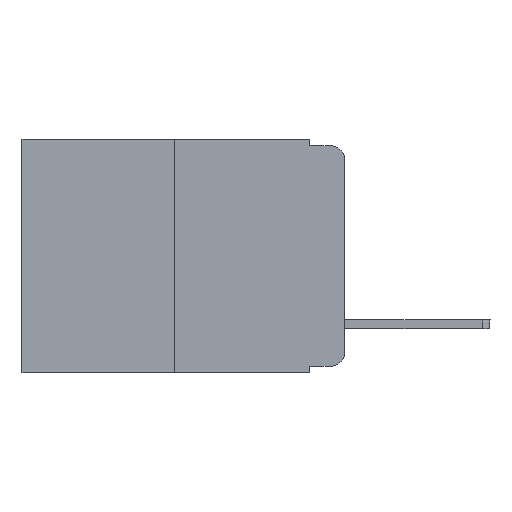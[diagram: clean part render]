
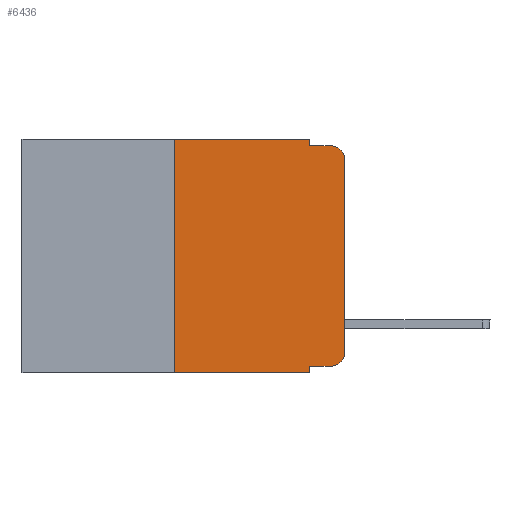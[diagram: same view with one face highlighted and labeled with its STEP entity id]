
A CAD part, left-side view. The second image highlights one B-rep face of the part: STEP entity #6436.
In plain terms, the highlighted planar face has unit normal (-1, 0, 0).
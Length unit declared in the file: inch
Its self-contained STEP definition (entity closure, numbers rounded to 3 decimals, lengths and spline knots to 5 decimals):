
#295 = LINE ( 'NONE', #18152, #21118 ) ;
#316 = VECTOR ( 'NONE', #17345, 39.37008 ) ;
#908 = VERTEX_POINT ( 'NONE', #2108 ) ;
#1001 = ORIENTED_EDGE ( 'NONE', *, *, #9225, .T. ) ;
#1073 = EDGE_CURVE ( 'NONE', #2855, #908, #17449, .T. ) ;
#1702 = DIRECTION ( 'NONE',  ( 0., -1., 0. ) ) ;
#1844 = VECTOR ( 'NONE', #20724, 39.37008 ) ;
#1947 = DIRECTION ( 'NONE',  ( 0., -1., 0. ) ) ;
#2108 = CARTESIAN_POINT ( 'NONE',  ( 0., 0.02, -0.333 ) ) ;
#2473 = CARTESIAN_POINT ( 'NONE',  ( 0., 0., -0.03 ) ) ;
#2579 = ORIENTED_EDGE ( 'NONE', *, *, #15121, .F. ) ;
#2637 = CARTESIAN_POINT ( 'NONE',  ( 0., 0.051, 0. ) ) ;
#2855 = VERTEX_POINT ( 'NONE', #9663 ) ;
#3003 = DIRECTION ( 'NONE',  ( 0., 0., -1. ) ) ;
#3525 = VECTOR ( 'NONE', #1947, 39.37008 ) ;
#3633 = AXIS2_PLACEMENT_3D ( 'NONE', #6027, #19022, #9798 ) ;
#4241 = LINE ( 'NONE', #8364, #20992 ) ;
#4399 = LINE ( 'NONE', #23824, #7563 ) ;
#4755 = EDGE_CURVE ( 'NONE', #8837, #4920, #20600, .T. ) ;
#4906 = EDGE_LOOP ( 'NONE', ( #14602, #11863, #21933, #11710, #2579, #14333, #6421, #10864, #15119, #1001 ) ) ;
#4920 = VERTEX_POINT ( 'NONE', #11579 ) ;
#4939 = DIRECTION ( 'NONE',  ( 0., 0., 1. ) ) ;
#5621 = EDGE_CURVE ( 'NONE', #19535, #14723, #4399, .T. ) ;
#6027 = CARTESIAN_POINT ( 'NONE',  ( 0., 0.02, -0.03 ) ) ;
#6421 = ORIENTED_EDGE ( 'NONE', *, *, #5621, .T. ) ;
#6436 = ADVANCED_FACE ( 'NONE', ( #19042 ), #17907, .F. ) ;
#6632 = CARTESIAN_POINT ( 'NONE',  ( 0., 0.051, 0. ) ) ;
#6854 = DIRECTION ( 'NONE',  ( 0., 0., 1. ) ) ;
#7078 = CARTESIAN_POINT ( 'NONE',  ( 0., 0.473, 0. ) ) ;
#7441 = CARTESIAN_POINT ( 'NONE',  ( 0., 0.051, -0.01 ) ) ;
#7563 = VECTOR ( 'NONE', #1702, 39.37008 ) ;
#7900 = VERTEX_POINT ( 'NONE', #21560 ) ;
#7903 = CARTESIAN_POINT ( 'NONE',  ( 0., 0.051, -0.333 ) ) ;
#7922 = CARTESIAN_POINT ( 'NONE',  ( 0., 0.051, 0. ) ) ;
#8364 = CARTESIAN_POINT ( 'NONE',  ( 0., 0.25, 0. ) ) ;
#8837 = VERTEX_POINT ( 'NONE', #15466 ) ;
#9062 = EDGE_CURVE ( 'NONE', #19535, #14202, #4241, .T. ) ;
#9225 = EDGE_CURVE ( 'NONE', #908, #7900, #19522, .T. ) ;
#9314 = CIRCLE ( 'NONE', #3633, 0.02 ) ;
#9467 = DIRECTION ( 'NONE',  ( 0., -1., 0. ) ) ;
#9663 = CARTESIAN_POINT ( 'NONE',  ( 0., 0.051, -0.333 ) ) ;
#9734 = CARTESIAN_POINT ( 'NONE',  ( 0., 0.051, -0.343 ) ) ;
#9798 = DIRECTION ( 'NONE',  ( 0., 0., -1. ) ) ;
#10069 = EDGE_CURVE ( 'NONE', #22306, #8837, #16290, .T. ) ;
#10257 = VECTOR ( 'NONE', #3003, 39.37008 ) ;
#10864 = ORIENTED_EDGE ( 'NONE', *, *, #21099, .F. ) ;
#11579 = CARTESIAN_POINT ( 'NONE',  ( 0., 0.02, -0.01 ) ) ;
#11710 = ORIENTED_EDGE ( 'NONE', *, *, #10069, .F. ) ;
#11863 = ORIENTED_EDGE ( 'NONE', *, *, #13498, .T. ) ;
#12086 = AXIS2_PLACEMENT_3D ( 'NONE', #13020, #14904, #18615 ) ;
#12912 = LINE ( 'NONE', #7078, #14690 ) ;
#12913 = CARTESIAN_POINT ( 'NONE',  ( 0., 0.25, -0.343 ) ) ;
#13020 = CARTESIAN_POINT ( 'NONE',  ( 0., 0.02, -0.313 ) ) ;
#13034 = DIRECTION ( 'NONE',  ( 0., 0., -1. ) ) ;
#13498 = EDGE_CURVE ( 'NONE', #22478, #4920, #9314, .T. ) ;
#14202 = VERTEX_POINT ( 'NONE', #23356 ) ;
#14333 = ORIENTED_EDGE ( 'NONE', *, *, #9062, .F. ) ;
#14602 = ORIENTED_EDGE ( 'NONE', *, *, #22064, .T. ) ;
#14690 = VECTOR ( 'NONE', #9467, 39.37008 ) ;
#14723 = VERTEX_POINT ( 'NONE', #9734 ) ;
#14904 = DIRECTION ( 'NONE',  ( -1., 0., 0. ) ) ;
#15119 = ORIENTED_EDGE ( 'NONE', *, *, #1073, .T. ) ;
#15121 = EDGE_CURVE ( 'NONE', #14202, #22306, #12912, .T. ) ;
#15466 = CARTESIAN_POINT ( 'NONE',  ( 0., 0.051, -0.01 ) ) ;
#16290 = LINE ( 'NONE', #6632, #10257 ) ;
#16292 = DIRECTION ( 'NONE',  ( 1., 0., 0. ) ) ;
#17345 = DIRECTION ( 'NONE',  ( 0., 0., -1. ) ) ;
#17449 = LINE ( 'NONE', #7903, #1844 ) ;
#17489 = CARTESIAN_POINT ( 'NONE',  ( 0., 0.473, 0. ) ) ;
#17907 = PLANE ( 'NONE',  #19885 ) ;
#18152 = CARTESIAN_POINT ( 'NONE',  ( 0., 0., 0. ) ) ;
#18615 = DIRECTION ( 'NONE',  ( 0., 0., -1. ) ) ;
#19022 = DIRECTION ( 'NONE',  ( -1., 0., 0. ) ) ;
#19042 = FACE_OUTER_BOUND ( 'NONE', #4906, .T. ) ;
#19522 = CIRCLE ( 'NONE', #12086, 0.02 ) ;
#19535 = VERTEX_POINT ( 'NONE', #12913 ) ;
#19885 = AXIS2_PLACEMENT_3D ( 'NONE', #17489, #16292, #13034 ) ;
#20600 = LINE ( 'NONE', #7441, #3525 ) ;
#20724 = DIRECTION ( 'NONE',  ( 0., -1., 0. ) ) ;
#20992 = VECTOR ( 'NONE', #4939, 39.37008 ) ;
#21099 = EDGE_CURVE ( 'NONE', #2855, #14723, #21407, .T. ) ;
#21118 = VECTOR ( 'NONE', #6854, 39.37008 ) ;
#21407 = LINE ( 'NONE', #2637, #316 ) ;
#21560 = CARTESIAN_POINT ( 'NONE',  ( 0., 0., -0.313 ) ) ;
#21933 = ORIENTED_EDGE ( 'NONE', *, *, #4755, .F. ) ;
#22064 = EDGE_CURVE ( 'NONE', #7900, #22478, #295, .T. ) ;
#22306 = VERTEX_POINT ( 'NONE', #7922 ) ;
#22478 = VERTEX_POINT ( 'NONE', #2473 ) ;
#23356 = CARTESIAN_POINT ( 'NONE',  ( 0., 0.25, 0. ) ) ;
#23824 = CARTESIAN_POINT ( 'NONE',  ( 0., 0.473, -0.343 ) ) ;
